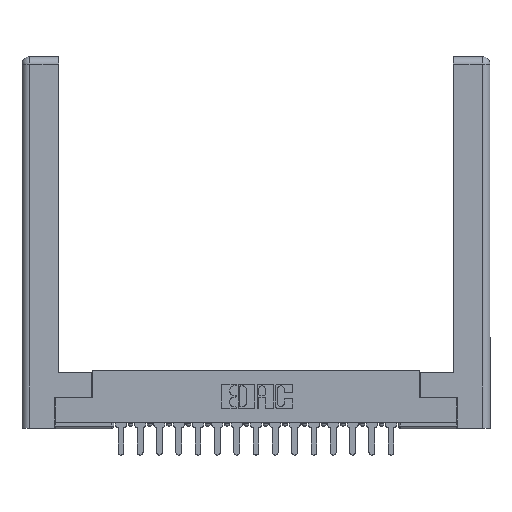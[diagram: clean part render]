
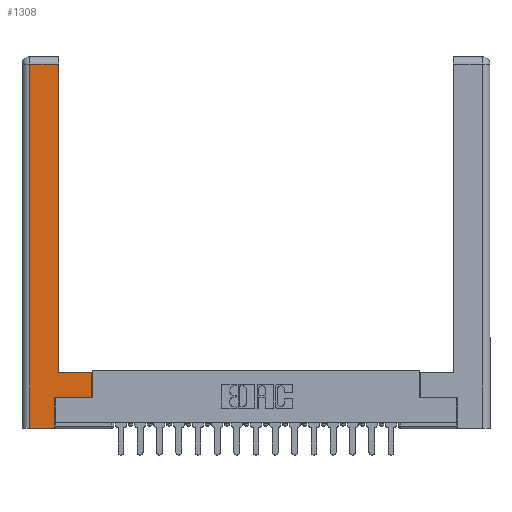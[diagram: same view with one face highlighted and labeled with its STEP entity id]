
A CAD part, top view. The second image highlights one B-rep face of the part: STEP entity #1308.
In plain terms, the highlighted planar face has unit normal (0, 0, 1).
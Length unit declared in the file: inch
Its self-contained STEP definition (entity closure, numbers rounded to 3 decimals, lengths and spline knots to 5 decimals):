
#30 = CARTESIAN_POINT ( 'NONE',  ( 0.265, 0.245, 0. ) ) ;
#121 = ORIENTED_EDGE ( 'NONE', *, *, #10825, .T. ) ;
#465 = LINE ( 'NONE', #13481, #3568 ) ;
#1308 = ADVANCED_FACE ( 'NONE', ( #15149 ), #6812, .F. ) ;
#1710 = VECTOR ( 'NONE', #13305, 39.37008 ) ;
#1941 = DIRECTION ( 'NONE',  ( -1., 0., 0. ) ) ;
#1993 = ORIENTED_EDGE ( 'NONE', *, *, #9969, .T. ) ;
#2039 = CARTESIAN_POINT ( 'NONE',  ( 0.295, 0.45, 0. ) ) ;
#2249 = VECTOR ( 'NONE', #11915, 39.37008 ) ;
#2318 = DIRECTION ( 'NONE',  ( 0., -1., 0. ) ) ;
#2321 = EDGE_CURVE ( 'NONE', #12697, #8455, #6788, .T. ) ;
#2483 = VECTOR ( 'NONE', #1941, 39.37008 ) ;
#2610 = ORIENTED_EDGE ( 'NONE', *, *, #2321, .T. ) ;
#2668 = VERTEX_POINT ( 'NONE', #17525 ) ;
#2991 = DIRECTION ( 'NONE',  ( 0., 1., 0. ) ) ;
#3104 = DIRECTION ( 'NONE',  ( 0., 1., 0. ) ) ;
#3452 = EDGE_CURVE ( 'NONE', #8455, #9382, #11562, .T. ) ;
#3464 = VECTOR ( 'NONE', #2991, 39.37008 ) ;
#3568 = VECTOR ( 'NONE', #6185, 39.37008 ) ;
#3786 = VERTEX_POINT ( 'NONE', #6384 ) ;
#4365 = DIRECTION ( 'NONE',  ( 1., 0., 0. ) ) ;
#4696 = AXIS2_PLACEMENT_3D ( 'NONE', #10972, #18202, #14108 ) ;
#4701 = LINE ( 'NONE', #30, #3464 ) ;
#5071 = VECTOR ( 'NONE', #3104, 39.37008 ) ;
#5620 = VECTOR ( 'NONE', #4365, 39.37008 ) ;
#5653 = VECTOR ( 'NONE', #2318, 39.37008 ) ;
#5849 = EDGE_CURVE ( 'NONE', #3786, #11908, #465, .T. ) ;
#6185 = DIRECTION ( 'NONE',  ( 0., 1., 0. ) ) ;
#6384 = CARTESIAN_POINT ( 'NONE',  ( 0.565, 0.245, 0. ) ) ;
#6788 = LINE ( 'NONE', #18379, #5653 ) ;
#6812 = PLANE ( 'NONE',  #4696 ) ;
#7548 = CARTESIAN_POINT ( 'NONE',  ( 0.0615, 0., 0. ) ) ;
#8097 = EDGE_CURVE ( 'NONE', #2668, #3786, #17378, .T. ) ;
#8455 = VERTEX_POINT ( 'NONE', #7548 ) ;
#8467 = EDGE_CURVE ( 'NONE', #9382, #2668, #4701, .T. ) ;
#8545 = CARTESIAN_POINT ( 'NONE',  ( 0.565, 0.45, 0. ) ) ;
#9220 = CARTESIAN_POINT ( 'NONE',  ( 0.0615, 2.94, 0. ) ) ;
#9382 = VERTEX_POINT ( 'NONE', #17736 ) ;
#9969 = EDGE_CURVE ( 'NONE', #13922, #12697, #11880, .T. ) ;
#10020 = CARTESIAN_POINT ( 'NONE',  ( 0.295, 2.94, 0. ) ) ;
#10098 = ORIENTED_EDGE ( 'NONE', *, *, #8467, .T. ) ;
#10511 = CARTESIAN_POINT ( 'NONE',  ( 0.295, 3., 0. ) ) ;
#10682 = LINE ( 'NONE', #2039, #2483 ) ;
#10825 = EDGE_CURVE ( 'NONE', #14483, #13922, #16395, .T. ) ;
#10972 = CARTESIAN_POINT ( 'NONE',  ( 0., 0., 0. ) ) ;
#11498 = CARTESIAN_POINT ( 'NONE',  ( 0.295, 0.45, 0. ) ) ;
#11562 = LINE ( 'NONE', #17386, #5620 ) ;
#11880 = LINE ( 'NONE', #9220, #1710 ) ;
#11908 = VERTEX_POINT ( 'NONE', #8545 ) ;
#11915 = DIRECTION ( 'NONE',  ( 1., 0., 0. ) ) ;
#12314 = EDGE_LOOP ( 'NONE', ( #121, #1993, #2610, #17488, #10098, #14242, #14538, #16385 ) ) ;
#12697 = VERTEX_POINT ( 'NONE', #16963 ) ;
#13305 = DIRECTION ( 'NONE',  ( -1., 0., 0. ) ) ;
#13481 = CARTESIAN_POINT ( 'NONE',  ( 0.565, 0.45, 0. ) ) ;
#13922 = VERTEX_POINT ( 'NONE', #10020 ) ;
#14108 = DIRECTION ( 'NONE',  ( -1., 0., 0. ) ) ;
#14242 = ORIENTED_EDGE ( 'NONE', *, *, #8097, .T. ) ;
#14483 = VERTEX_POINT ( 'NONE', #11498 ) ;
#14538 = ORIENTED_EDGE ( 'NONE', *, *, #5849, .T. ) ;
#15149 = FACE_OUTER_BOUND ( 'NONE', #12314, .T. ) ;
#16028 = CARTESIAN_POINT ( 'NONE',  ( 0.565, 0.245, 0. ) ) ;
#16385 = ORIENTED_EDGE ( 'NONE', *, *, #16779, .T. ) ;
#16395 = LINE ( 'NONE', #10511, #5071 ) ;
#16779 = EDGE_CURVE ( 'NONE', #11908, #14483, #10682, .T. ) ;
#16963 = CARTESIAN_POINT ( 'NONE',  ( 0.0615, 2.94, 0. ) ) ;
#17378 = LINE ( 'NONE', #16028, #2249 ) ;
#17386 = CARTESIAN_POINT ( 'NONE',  ( 0.265, 0., 0. ) ) ;
#17488 = ORIENTED_EDGE ( 'NONE', *, *, #3452, .T. ) ;
#17525 = CARTESIAN_POINT ( 'NONE',  ( 0.265, 0.245, 0. ) ) ;
#17736 = CARTESIAN_POINT ( 'NONE',  ( 0.265, 0., 0. ) ) ;
#18202 = DIRECTION ( 'NONE',  ( 0., 0., -1. ) ) ;
#18379 = CARTESIAN_POINT ( 'NONE',  ( 0.0615, 0., 0. ) ) ;
